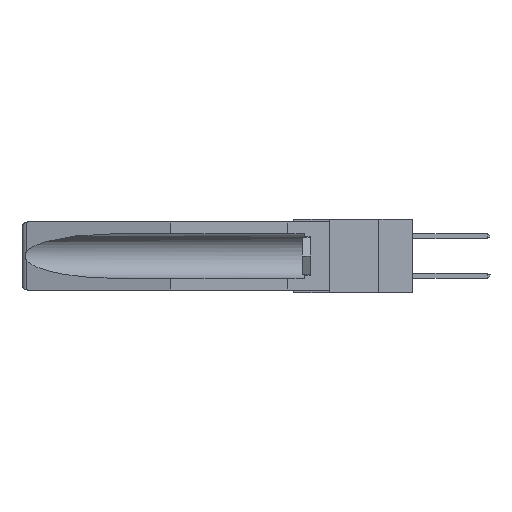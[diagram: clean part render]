
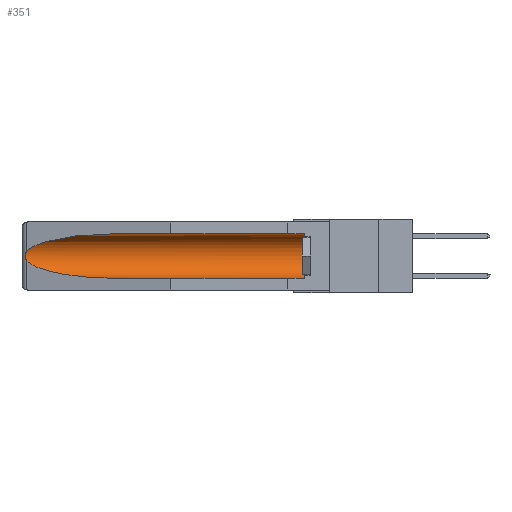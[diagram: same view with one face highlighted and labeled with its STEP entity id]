
A CAD part, left-side view. The second image highlights one B-rep face of the part: STEP entity #351.
In plain terms, the highlighted cylindrical face has radius 2.857 mm (diameter 5.715 mm), a partial arc.
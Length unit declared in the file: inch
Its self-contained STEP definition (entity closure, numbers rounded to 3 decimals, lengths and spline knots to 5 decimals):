
#47 = CARTESIAN_POINT ( 'NONE',  ( 0.26655, 1.53094, -0.18657 ) ) ;
#150 = VECTOR ( 'NONE', #17129, 39.37008 ) ;
#247 = EDGE_CURVE ( 'NONE', #13394, #5829, #11401, .T. ) ;
#351 = ADVANCED_FACE ( 'NONE', ( #595 ), #18759, .F. ) ;
#557 = CARTESIAN_POINT ( 'NONE',  ( 0.25451, 1.48313, -0.24835 ) ) ;
#595 = FACE_OUTER_BOUND ( 'NONE', #8629, .T. ) ;
#721 = ORIENTED_EDGE ( 'NONE', *, *, #10766, .F. ) ;
#1284 = CIRCLE ( 'NONE', #11510, 0.1125 ) ;
#1694 = ORIENTED_EDGE ( 'NONE', *, *, #14329, .T. ) ;
#1709 = CARTESIAN_POINT ( 'NONE',  ( 0.21114, 1.30732, -0.284 ) ) ;
#2352 = B_SPLINE_CURVE_WITH_KNOTS ( 'NONE', 3,
 ( #15019, #7740, #9208, #4835, #7440, #11726, #17719, #47, #11619, #8732 ),
 .UNSPECIFIED., .F., .F.,
 ( 4, 2, 2, 2, 4 ),
 ( 0., 0.00029, 0.00058, 0.00087, 0.00117 ),
 .UNSPECIFIED. ) ;
#2772 = CARTESIAN_POINT ( 'NONE',  ( 0.25451, 1.48313, -0.09465 ) ) ;
#3811 = CARTESIAN_POINT ( 'NONE',  ( 0.155, -0.30754, -0.284 ) ) ;
#3932 = CARTESIAN_POINT ( 'NONE',  ( 0.155, -0.30754, -0.059 ) ) ;
#4735 = VECTOR ( 'NONE', #6790, 39.37008 ) ;
#4835 = CARTESIAN_POINT ( 'NONE',  ( 0.2673, 1.5327, -0.16383 ) ) ;
#5744 = CARTESIAN_POINT ( 'NONE',  ( 0.26537, 1.52718, -0.14972 ) ) ;
#5829 = VERTEX_POINT ( 'NONE', #12875 ) ;
#6162 = CARTESIAN_POINT ( 'NONE',  ( 0.155, 1.07973, -0.284 ) ) ;
#6294 = CARTESIAN_POINT ( 'NONE',  ( 0.26537, 1.52718, -0.19328 ) ) ;
#6311 = EDGE_CURVE ( 'NONE', #9947, #9440, #2352, .T. ) ;
#6536 = AXIS2_PLACEMENT_3D ( 'NONE', #14513, #7215, #10095 ) ;
#6790 = DIRECTION ( 'NONE',  ( 0., 1., 0. ) ) ;
#7100 = CARTESIAN_POINT ( 'NONE',  ( 0.26537, 1.52718, -0.19328 ) ) ;
#7215 = DIRECTION ( 'NONE',  ( 0., 1., 0. ) ) ;
#7440 = CARTESIAN_POINT ( 'NONE',  ( 0.2675, 1.53308, -0.16763 ) ) ;
#7551 = VERTEX_POINT ( 'NONE', #15802 ) ;
#7740 = CARTESIAN_POINT ( 'NONE',  ( 0.26597, 1.52961, -0.15275 ) ) ;
#8193 =( BOUNDED_CURVE ( )  B_SPLINE_CURVE ( 3, ( #17121, #18613, #2772, #5744 ),
 .UNSPECIFIED., .F., .T. ) 
 B_SPLINE_CURVE_WITH_KNOTS ( ( 4, 4 ),
 ( 4.71239, 6.08839 ),
 .UNSPECIFIED. ) 
 CURVE ( )  GEOMETRIC_REPRESENTATION_ITEM ( )  RATIONAL_B_SPLINE_CURVE ( ( 1., 0.848, 0.848, 1. ) ) 
 REPRESENTATION_ITEM ( '' )  );
#8629 = EDGE_LOOP ( 'NONE', ( #11548, #10479, #12328, #721, #1694, #9469 ) ) ;
#8732 = CARTESIAN_POINT ( 'NONE',  ( 0.26537, 1.52718, -0.19328 ) ) ;
#9208 = CARTESIAN_POINT ( 'NONE',  ( 0.26654, 1.53092, -0.15636 ) ) ;
#9440 = VERTEX_POINT ( 'NONE', #7100 ) ;
#9469 = ORIENTED_EDGE ( 'NONE', *, *, #247, .T. ) ;
#9603 = CARTESIAN_POINT ( 'NONE',  ( 0.155, 0.126, -0.059 ) ) ;
#9947 = VERTEX_POINT ( 'NONE', #10652 ) ;
#10095 = DIRECTION ( 'NONE',  ( 0., 0., 1. ) ) ;
#10479 = ORIENTED_EDGE ( 'NONE', *, *, #6311, .T. ) ;
#10652 = CARTESIAN_POINT ( 'NONE',  ( 0.26537, 1.52718, -0.14972 ) ) ;
#10766 = EDGE_CURVE ( 'NONE', #7551, #14042, #18360, .T. ) ;
#10973 =( BOUNDED_CURVE ( )  B_SPLINE_CURVE ( 3, ( #6294, #557, #1709, #6162 ),
 .UNSPECIFIED., .F., .F. ) 
 B_SPLINE_CURVE_WITH_KNOTS ( ( 4, 4 ),
 ( 0.1948, 1.5708 ),
 .UNSPECIFIED. ) 
 CURVE ( )  GEOMETRIC_REPRESENTATION_ITEM ( )  RATIONAL_B_SPLINE_CURVE ( ( 1., 0.848, 0.848, 1. ) ) 
 REPRESENTATION_ITEM ( '' )  );
#11019 = CARTESIAN_POINT ( 'NONE',  ( 0.155, 0.126, -0.1715 ) ) ;
#11401 = LINE ( 'NONE', #3932, #4735 ) ;
#11510 = AXIS2_PLACEMENT_3D ( 'NONE', #11019, #13085, #13857 ) ;
#11548 = ORIENTED_EDGE ( 'NONE', *, *, #18761, .T. ) ;
#11619 = CARTESIAN_POINT ( 'NONE',  ( 0.26597, 1.5296, -0.19026 ) ) ;
#11726 = CARTESIAN_POINT ( 'NONE',  ( 0.2675, 1.53308, -0.17534 ) ) ;
#11776 = EDGE_CURVE ( 'NONE', #9440, #14042, #10973, .T. ) ;
#12328 = ORIENTED_EDGE ( 'NONE', *, *, #11776, .T. ) ;
#12875 = CARTESIAN_POINT ( 'NONE',  ( 0.155, 1.07973, -0.059 ) ) ;
#13085 = DIRECTION ( 'NONE',  ( 0., -1., 0. ) ) ;
#13394 = VERTEX_POINT ( 'NONE', #9603 ) ;
#13857 = DIRECTION ( 'NONE',  ( 0., 0., 1. ) ) ;
#14042 = VERTEX_POINT ( 'NONE', #15488 ) ;
#14329 = EDGE_CURVE ( 'NONE', #7551, #13394, #1284, .T. ) ;
#14513 = CARTESIAN_POINT ( 'NONE',  ( 0.155, -0.30754, -0.1715 ) ) ;
#15019 = CARTESIAN_POINT ( 'NONE',  ( 0.26537, 1.52718, -0.14972 ) ) ;
#15488 = CARTESIAN_POINT ( 'NONE',  ( 0.155, 1.07973, -0.284 ) ) ;
#15802 = CARTESIAN_POINT ( 'NONE',  ( 0.155, 0.126, -0.284 ) ) ;
#17121 = CARTESIAN_POINT ( 'NONE',  ( 0.155, 1.07973, -0.059 ) ) ;
#17129 = DIRECTION ( 'NONE',  ( 0., 1., 0. ) ) ;
#17719 = CARTESIAN_POINT ( 'NONE',  ( 0.2673, 1.53269, -0.17917 ) ) ;
#18360 = LINE ( 'NONE', #3811, #150 ) ;
#18613 = CARTESIAN_POINT ( 'NONE',  ( 0.21114, 1.30732, -0.059 ) ) ;
#18759 = CYLINDRICAL_SURFACE ( 'NONE', #6536, 0.1125 ) ;
#18761 = EDGE_CURVE ( 'NONE', #5829, #9947, #8193, .T. ) ;
